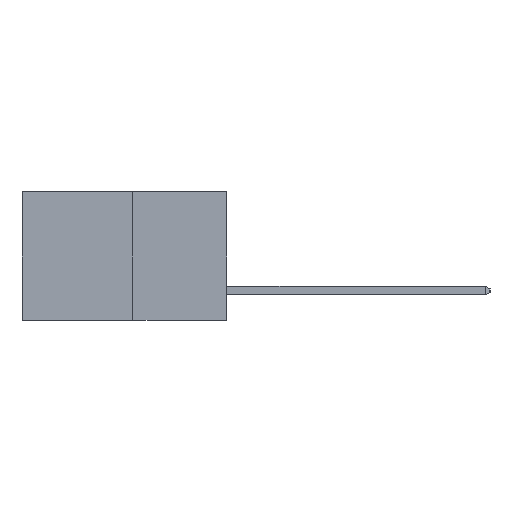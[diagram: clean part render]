
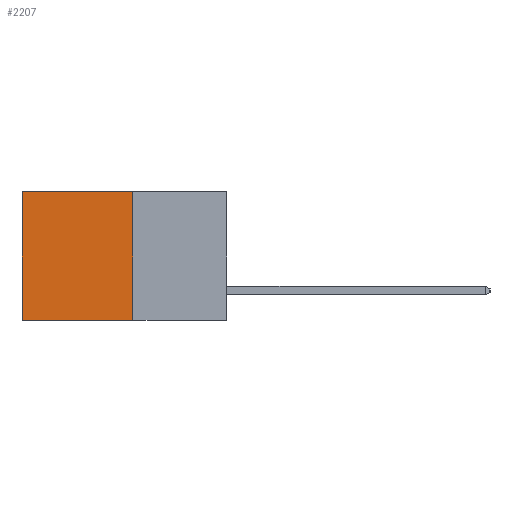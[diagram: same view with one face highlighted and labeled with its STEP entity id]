
A CAD part, left-side view. The second image highlights one B-rep face of the part: STEP entity #2207.
In plain terms, the highlighted planar face has unit normal (-1, 0, 0).
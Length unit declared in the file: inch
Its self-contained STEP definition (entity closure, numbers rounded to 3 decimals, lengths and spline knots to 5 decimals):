
#1068 = EDGE_CURVE ( 'NONE', #15124, #5162, #11829, .T. ) ;
#1154 = LINE ( 'NONE', #6599, #10235 ) ;
#1326 = VERTEX_POINT ( 'NONE', #2721 ) ;
#1613 = CARTESIAN_POINT ( 'NONE',  ( 0.277, 0.27, -0.37 ) ) ;
#2073 = FACE_OUTER_BOUND ( 'NONE', #5075, .T. ) ;
#2207 = ADVANCED_FACE ( 'NONE', ( #2073 ), #7599, .F. ) ;
#2568 = ORIENTED_EDGE ( 'NONE', *, *, #1068, .F. ) ;
#2721 = CARTESIAN_POINT ( 'NONE',  ( 0.277, 0.59, 0. ) ) ;
#5075 = EDGE_LOOP ( 'NONE', ( #12348, #7129, #2568, #11476 ) ) ;
#5162 = VERTEX_POINT ( 'NONE', #9842 ) ;
#5382 = EDGE_CURVE ( 'NONE', #5162, #15393, #1154, .T. ) ;
#5513 = LINE ( 'NONE', #10300, #14845 ) ;
#6245 = AXIS2_PLACEMENT_3D ( 'NONE', #7246, #7548, #13088 ) ;
#6599 = CARTESIAN_POINT ( 'NONE',  ( 0.277, 0.27, -0.37 ) ) ;
#6872 = DIRECTION ( 'NONE',  ( 0., 0., -1. ) ) ;
#7129 = ORIENTED_EDGE ( 'NONE', *, *, #5382, .F. ) ;
#7246 = CARTESIAN_POINT ( 'NONE',  ( 0.277, 0.27, -0.37 ) ) ;
#7548 = DIRECTION ( 'NONE',  ( 1., 0., 0. ) ) ;
#7599 = PLANE ( 'NONE',  #6245 ) ;
#7608 = LINE ( 'NONE', #14900, #10466 ) ;
#8159 = VECTOR ( 'NONE', #6872, 39.37008 ) ;
#8393 = EDGE_CURVE ( 'NONE', #15124, #1326, #5513, .T. ) ;
#8747 = CARTESIAN_POINT ( 'NONE',  ( 0.277, 0.27, 0. ) ) ;
#8837 = DIRECTION ( 'NONE',  ( 0., 0., -1. ) ) ;
#8942 = EDGE_CURVE ( 'NONE', #1326, #15393, #7608, .T. ) ;
#9044 = DIRECTION ( 'NONE',  ( 0., 1., 0. ) ) ;
#9080 = DIRECTION ( 'NONE',  ( 0., 1., 0. ) ) ;
#9239 = CARTESIAN_POINT ( 'NONE',  ( 0.277, 0.59, -0.37 ) ) ;
#9842 = CARTESIAN_POINT ( 'NONE',  ( 0.277, 0.27, -0.37 ) ) ;
#10235 = VECTOR ( 'NONE', #9044, 39.37008 ) ;
#10300 = CARTESIAN_POINT ( 'NONE',  ( 0.277, 0.27, 0. ) ) ;
#10466 = VECTOR ( 'NONE', #8837, 39.37008 ) ;
#11476 = ORIENTED_EDGE ( 'NONE', *, *, #8393, .T. ) ;
#11829 = LINE ( 'NONE', #1613, #8159 ) ;
#12348 = ORIENTED_EDGE ( 'NONE', *, *, #8942, .T. ) ;
#13088 = DIRECTION ( 'NONE',  ( 0., 0., -1. ) ) ;
#14845 = VECTOR ( 'NONE', #9080, 39.37008 ) ;
#14900 = CARTESIAN_POINT ( 'NONE',  ( 0.277, 0.59, -0.37 ) ) ;
#15124 = VERTEX_POINT ( 'NONE', #8747 ) ;
#15393 = VERTEX_POINT ( 'NONE', #9239 ) ;
